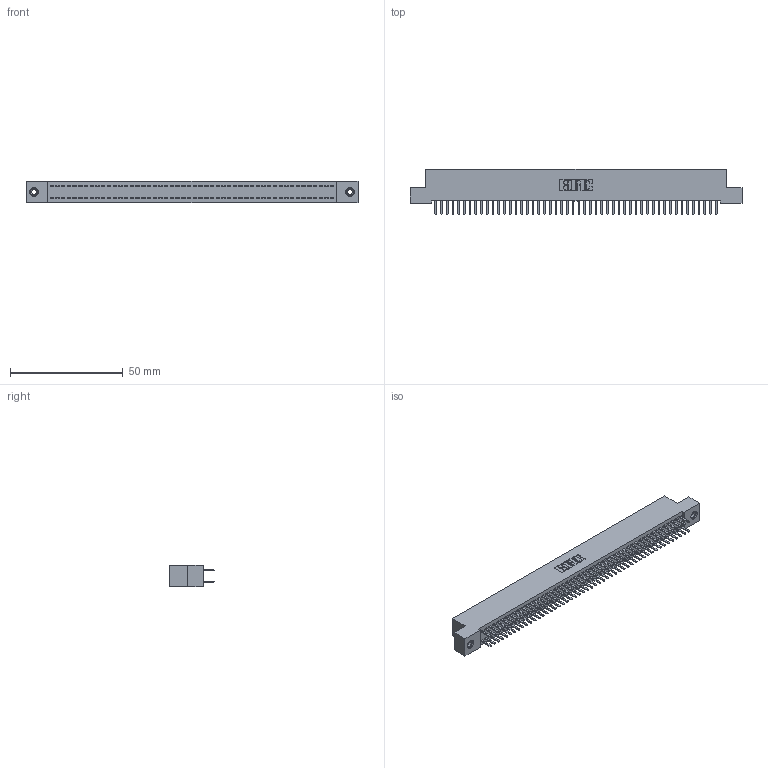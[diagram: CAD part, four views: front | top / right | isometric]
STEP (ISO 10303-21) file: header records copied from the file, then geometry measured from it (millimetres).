
FILE_DESCRIPTION (( 'STEP AP203' ), '1' );
FILE_NAME ('392-100-520-208.STEP', '2019-10-09T20:42:16', ( '' ), ( '' ), 'SwSTEP 2.0', 'SolidWorks 2016', '' );
FILE_SCHEMA (( 'CONFIG_CONTROL_DESIGN' ));
Length unit declared in the file: inch
Products named in the file (4): 345-292-001_345-293-120; 345-250-001_345-250-003-102; 392-100-520-208; 342 Part_TI
Assembly tree (103 placements, depth 2):
  392-100-520-208
    342 Part_TI
    345-292-001_345-293-120  x100
    345-250-001_345-250-003-102  x2
Bounding box: 147.32 x 20.02 x 9.4 mm (x, y, z)
Volume: 13224.9 mm3; surface area: 21630.5 mm2
Topology: 103 solids, 103 shells, 5770 faces, 16735 edges, 10882 vertices
Faces by surface type: plane 3898, cylinder 1856, cone 12, torus 4
Entity records: 32300 total; most frequent: CARTESIAN_POINT 5337, ORIENTED_EDGE 5254, DIRECTION 4565, EDGE_CURVE 2627, VECTOR 2475, LINE 2475, VERTEX_POINT 1744, AXIS2_PLACEMENT_3D 1045
